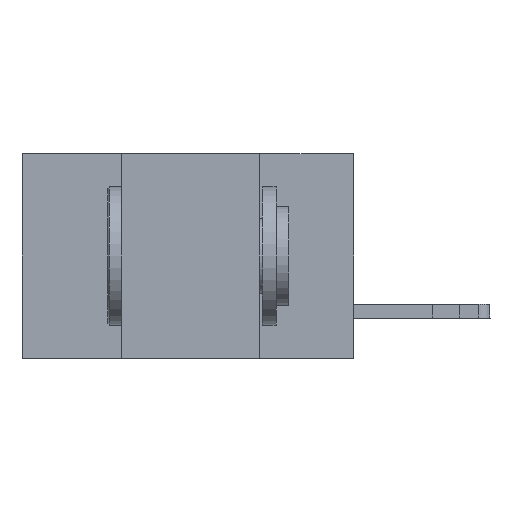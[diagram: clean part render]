
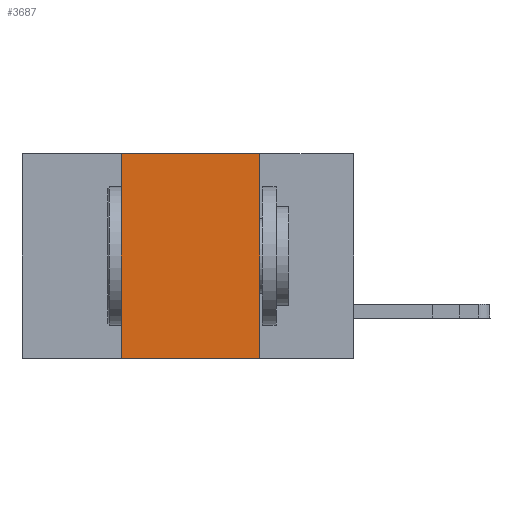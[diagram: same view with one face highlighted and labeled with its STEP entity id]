
A CAD part, left-side view. The second image highlights one B-rep face of the part: STEP entity #3687.
In plain terms, the highlighted planar face has unit normal (-1, 0, 0).
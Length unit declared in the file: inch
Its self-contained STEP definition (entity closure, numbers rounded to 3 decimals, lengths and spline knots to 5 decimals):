
#487 = DIRECTION ( 'NONE',  ( 0., 0., -1. ) ) ;
#1342 = EDGE_CURVE ( 'NONE', #5654, #19239, #21256, .T. ) ;
#1389 = ORIENTED_EDGE ( 'NONE', *, *, #7415, .F. ) ;
#2925 = VECTOR ( 'NONE', #487, 39.37008 ) ;
#3687 = ADVANCED_FACE ( 'NONE', ( #10405 ), #14021, .F. ) ;
#4154 = CARTESIAN_POINT ( 'NONE',  ( 0., 0.17, 0. ) ) ;
#4681 = DIRECTION ( 'NONE',  ( 0., -1., 0. ) ) ;
#5027 = AXIS2_PLACEMENT_3D ( 'NONE', #14152, #13602, #13524 ) ;
#5654 = VERTEX_POINT ( 'NONE', #4154 ) ;
#6665 = ORIENTED_EDGE ( 'NONE', *, *, #11237, .T. ) ;
#7229 = VECTOR ( 'NONE', #12312, 39.37008 ) ;
#7415 = EDGE_CURVE ( 'NONE', #7618, #5654, #9297, .T. ) ;
#7618 = VERTEX_POINT ( 'NONE', #15635 ) ;
#8326 = DIRECTION ( 'NONE',  ( 0., -1., 0. ) ) ;
#8533 = LINE ( 'NONE', #16880, #16560 ) ;
#9297 = LINE ( 'NONE', #21793, #12784 ) ;
#10405 = FACE_OUTER_BOUND ( 'NONE', #11047, .T. ) ;
#10585 = CARTESIAN_POINT ( 'NONE',  ( 0., 0.42, 0. ) ) ;
#11047 = EDGE_LOOP ( 'NONE', ( #13723, #1389, #16341, #6665 ) ) ;
#11237 = EDGE_CURVE ( 'NONE', #22310, #19239, #8533, .T. ) ;
#12312 = DIRECTION ( 'NONE',  ( 0., 0., 1. ) ) ;
#12585 = CARTESIAN_POINT ( 'NONE',  ( 0., 0.17, 0. ) ) ;
#12784 = VECTOR ( 'NONE', #4681, 39.37008 ) ;
#13524 = DIRECTION ( 'NONE',  ( 0., 0., -1. ) ) ;
#13602 = DIRECTION ( 'NONE',  ( 1., 0., 0. ) ) ;
#13723 = ORIENTED_EDGE ( 'NONE', *, *, #1342, .F. ) ;
#14021 = PLANE ( 'NONE',  #5027 ) ;
#14152 = CARTESIAN_POINT ( 'NONE',  ( 0., 0.6, 0. ) ) ;
#15114 = CARTESIAN_POINT ( 'NONE',  ( 0., 0.17, -0.37 ) ) ;
#15383 = EDGE_CURVE ( 'NONE', #22310, #7618, #21375, .T. ) ;
#15635 = CARTESIAN_POINT ( 'NONE',  ( 0., 0.42, 0. ) ) ;
#15931 = CARTESIAN_POINT ( 'NONE',  ( 0., 0.42, -0.37 ) ) ;
#16341 = ORIENTED_EDGE ( 'NONE', *, *, #15383, .F. ) ;
#16560 = VECTOR ( 'NONE', #8326, 39.37008 ) ;
#16880 = CARTESIAN_POINT ( 'NONE',  ( 0., 0.6, -0.37 ) ) ;
#19239 = VERTEX_POINT ( 'NONE', #15114 ) ;
#21256 = LINE ( 'NONE', #12585, #2925 ) ;
#21375 = LINE ( 'NONE', #10585, #7229 ) ;
#21793 = CARTESIAN_POINT ( 'NONE',  ( 0., 0.6, 0. ) ) ;
#22310 = VERTEX_POINT ( 'NONE', #15931 ) ;
